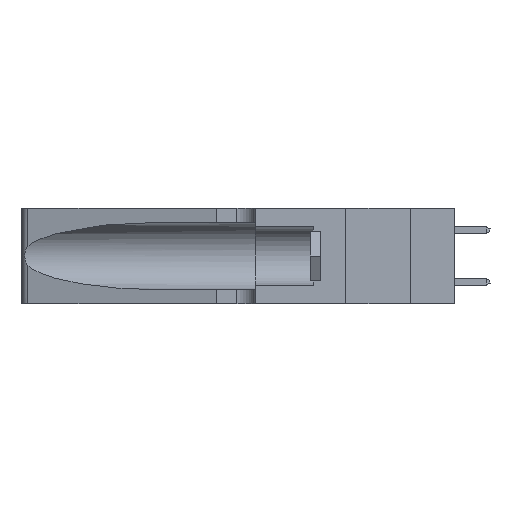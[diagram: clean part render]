
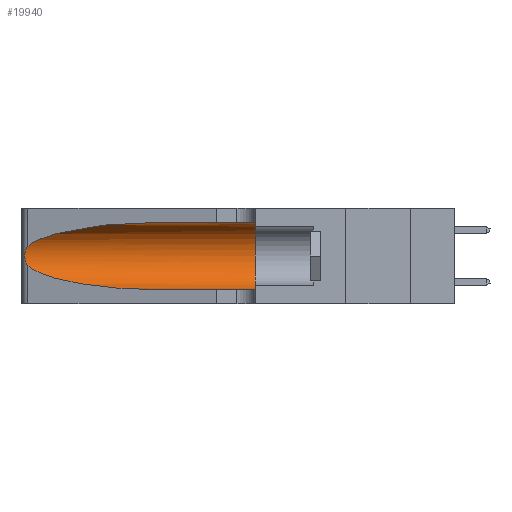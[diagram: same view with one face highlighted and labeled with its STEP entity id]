
A CAD part, left-side view. The second image highlights one B-rep face of the part: STEP entity #19940.
In plain terms, the highlighted cylindrical face has radius 3.308 mm (diameter 6.617 mm), a partial arc.
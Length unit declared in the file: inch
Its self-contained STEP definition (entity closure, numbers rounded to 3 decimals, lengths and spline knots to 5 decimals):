
#6 = CARTESIAN_POINT ( 'NONE',  ( 0.1305, 0.35, 0.31525 ) ) ;
#318 = AXIS2_PLACEMENT_3D ( 'NONE', #12591, #12365, #15178 ) ;
#681 = VERTEX_POINT ( 'NONE', #6 ) ;
#1166 = LINE ( 'NONE', #12852, #7979 ) ;
#1235 = CARTESIAN_POINT ( 'NONE',  ( 0.26075, 1.23896, 0.19203 ) ) ;
#2490 = B_SPLINE_CURVE_WITH_KNOTS ( 'NONE', 3,
 ( #20568, #29118, #26770, #8834, #6143, #11416, #1235, #3805, #27010, #31590, #29699, #17173, #19454, #6935 ),
 .UNSPECIFIED., .F., .F.,
 ( 4, 2, 2, 2, 2, 2, 4 ),
 ( 0., 0.00027, 0.00053, 0.00107, 0.0016, 0.00187, 0.00214 ),
 .UNSPECIFIED. ) ;
#3156 = CARTESIAN_POINT ( 'NONE',  ( 0.18966, 0.96281, 0.05475 ) ) ;
#3607 = EDGE_LOOP ( 'NONE', ( #22357, #31708, #7137, #19516, #8962, #10839 ) ) ;
#3805 = CARTESIAN_POINT ( 'NONE',  ( 0.26075, 1.23896, 0.178 ) ) ;
#5210 = CARTESIAN_POINT ( 'NONE',  ( 0.25487, 1.22718, 0.14631 ) ) ;
#5831 = CARTESIAN_POINT ( 'NONE',  ( 0.1305, 1.61858, 0.05475 ) ) ;
#5908 = DIRECTION ( 'NONE',  ( 0., -1., 0. ) ) ;
#6143 = CARTESIAN_POINT ( 'NONE',  ( 0.25854, 1.2359, 0.20912 ) ) ;
#6935 = CARTESIAN_POINT ( 'NONE',  ( 0.25487, 1.22718, 0.14631 ) ) ;
#7137 = ORIENTED_EDGE ( 'NONE', *, *, #17159, .T. ) ;
#7979 = VECTOR ( 'NONE', #30988, 39.37008 ) ;
#8372 =( BOUNDED_CURVE ( )  B_SPLINE_CURVE ( 3, ( #25592, #20325, #3156, #23639 ),
 .UNSPECIFIED., .F., .F. ) 
 B_SPLINE_CURVE_WITH_KNOTS ( ( 4, 4 ),
 ( 3.44316, 4.71239 ),
 .UNSPECIFIED. ) 
 CURVE ( )  GEOMETRIC_REPRESENTATION_ITEM ( )  RATIONAL_B_SPLINE_CURVE ( ( 1., 0.87, 0.87, 1. ) ) 
 REPRESENTATION_ITEM ( '' )  );
#8834 = CARTESIAN_POINT ( 'NONE',  ( 0.25787, 1.23484, 0.2124 ) ) ;
#8962 = ORIENTED_EDGE ( 'NONE', *, *, #26845, .F. ) ;
#10054 = VERTEX_POINT ( 'NONE', #31921 ) ;
#10839 = ORIENTED_EDGE ( 'NONE', *, *, #14583, .F. ) ;
#11170 = DIRECTION ( 'NONE',  ( 0., 0., -1. ) ) ;
#11416 = CARTESIAN_POINT ( 'NONE',  ( 0.26018, 1.23835, 0.19895 ) ) ;
#11659 = CARTESIAN_POINT ( 'NONE',  ( 0.1305, 0.72297, 0.31525 ) ) ;
#11931 = EDGE_CURVE ( 'NONE', #13793, #28014, #17299, .T. ) ;
#12365 = DIRECTION ( 'NONE',  ( 0., 1., 0. ) ) ;
#12491 = CARTESIAN_POINT ( 'NONE',  ( 0.1305, 0.72297, 0.31525 ) ) ;
#12591 = CARTESIAN_POINT ( 'NONE',  ( 0.1305, 0.35, 0.185 ) ) ;
#12852 = CARTESIAN_POINT ( 'NONE',  ( 0.1305, 1.61858, 0.31525 ) ) ;
#13793 = VERTEX_POINT ( 'NONE', #12491 ) ;
#14570 = CARTESIAN_POINT ( 'NONE',  ( 0.1305, 0.35, 0.05475 ) ) ;
#14583 = EDGE_CURVE ( 'NONE', #13793, #681, #1166, .T. ) ;
#15178 = DIRECTION ( 'NONE',  ( 0., 0., 1. ) ) ;
#17159 = EDGE_CURVE ( 'NONE', #17990, #10054, #8372, .T. ) ;
#17173 = CARTESIAN_POINT ( 'NONE',  ( 0.25639, 1.23186, 0.15144 ) ) ;
#17299 =( BOUNDED_CURVE ( )  B_SPLINE_CURVE ( 3, ( #11659, #24277, #32176, #26897 ),
 .UNSPECIFIED., .F., .F. ) 
 B_SPLINE_CURVE_WITH_KNOTS ( ( 4, 4 ),
 ( 1.5708, 2.84003 ),
 .UNSPECIFIED. ) 
 CURVE ( )  GEOMETRIC_REPRESENTATION_ITEM ( )  RATIONAL_B_SPLINE_CURVE ( ( 1., 0.87, 0.87, 1. ) ) 
 REPRESENTATION_ITEM ( '' )  );
#17672 = VECTOR ( 'NONE', #28803, 39.37008 ) ;
#17990 = VERTEX_POINT ( 'NONE', #5210 ) ;
#19454 = CARTESIAN_POINT ( 'NONE',  ( 0.25555, 1.22993, 0.14849 ) ) ;
#19516 = ORIENTED_EDGE ( 'NONE', *, *, #28655, .T. ) ;
#19940 = ADVANCED_FACE ( 'NONE', ( #28213 ), #32239, .F. ) ;
#20245 = VERTEX_POINT ( 'NONE', #14570 ) ;
#20325 = CARTESIAN_POINT ( 'NONE',  ( 0.2373, 1.15595, 0.08982 ) ) ;
#20539 = AXIS2_PLACEMENT_3D ( 'NONE', #20944, #5908, #11170 ) ;
#20568 = CARTESIAN_POINT ( 'NONE',  ( 0.25487, 1.22718, 0.22369 ) ) ;
#20944 = CARTESIAN_POINT ( 'NONE',  ( 0.1305, 1.61858, 0.185 ) ) ;
#22357 = ORIENTED_EDGE ( 'NONE', *, *, #11931, .T. ) ;
#23639 = CARTESIAN_POINT ( 'NONE',  ( 0.1305, 0.72297, 0.05475 ) ) ;
#24277 = CARTESIAN_POINT ( 'NONE',  ( 0.18966, 0.96281, 0.31525 ) ) ;
#24676 = EDGE_CURVE ( 'NONE', #28014, #17990, #2490, .T. ) ;
#25592 = CARTESIAN_POINT ( 'NONE',  ( 0.25487, 1.22718, 0.14631 ) ) ;
#26770 = CARTESIAN_POINT ( 'NONE',  ( 0.25639, 1.23184, 0.21858 ) ) ;
#26845 = EDGE_CURVE ( 'NONE', #681, #20245, #31178, .T. ) ;
#26897 = CARTESIAN_POINT ( 'NONE',  ( 0.25487, 1.22718, 0.22369 ) ) ;
#27010 = CARTESIAN_POINT ( 'NONE',  ( 0.26017, 1.23833, 0.17102 ) ) ;
#28014 = VERTEX_POINT ( 'NONE', #33118 ) ;
#28213 = FACE_OUTER_BOUND ( 'NONE', #3607, .T. ) ;
#28537 = LINE ( 'NONE', #5831, #17672 ) ;
#28655 = EDGE_CURVE ( 'NONE', #10054, #20245, #28537, .T. ) ;
#28803 = DIRECTION ( 'NONE',  ( 0., -1., 0. ) ) ;
#29118 = CARTESIAN_POINT ( 'NONE',  ( 0.25555, 1.22994, 0.2215 ) ) ;
#29699 = CARTESIAN_POINT ( 'NONE',  ( 0.25789, 1.23486, 0.15765 ) ) ;
#30988 = DIRECTION ( 'NONE',  ( 0., -1., 0. ) ) ;
#31178 = CIRCLE ( 'NONE', #318, 0.13025 ) ;
#31590 = CARTESIAN_POINT ( 'NONE',  ( 0.25856, 1.23593, 0.16098 ) ) ;
#31708 = ORIENTED_EDGE ( 'NONE', *, *, #24676, .T. ) ;
#31921 = CARTESIAN_POINT ( 'NONE',  ( 0.1305, 0.72297, 0.05475 ) ) ;
#32176 = CARTESIAN_POINT ( 'NONE',  ( 0.2373, 1.15595, 0.28018 ) ) ;
#32239 = CYLINDRICAL_SURFACE ( 'NONE', #20539, 0.13025 ) ;
#33118 = CARTESIAN_POINT ( 'NONE',  ( 0.25487, 1.22718, 0.22369 ) ) ;
